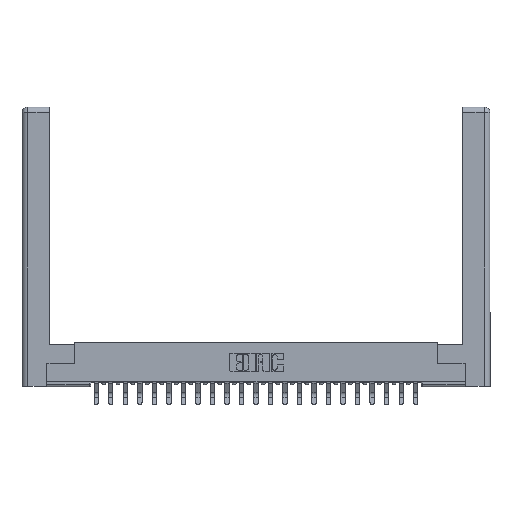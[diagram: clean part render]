
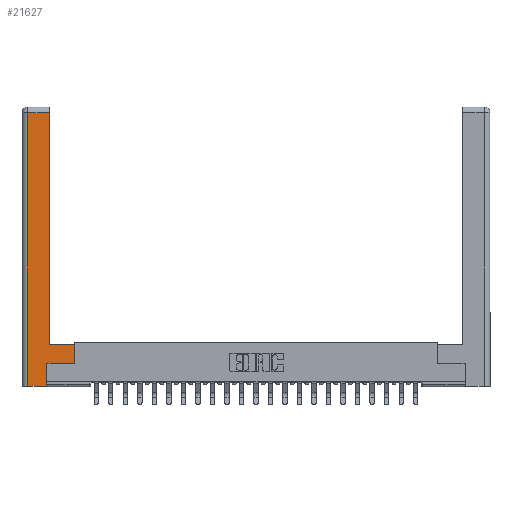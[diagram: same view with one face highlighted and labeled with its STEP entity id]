
A CAD part, top view. The second image highlights one B-rep face of the part: STEP entity #21627.
In plain terms, the highlighted planar face has unit normal (0, 0, 1).
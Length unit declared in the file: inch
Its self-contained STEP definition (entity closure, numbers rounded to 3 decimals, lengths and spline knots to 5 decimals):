
#479 = VECTOR ( 'NONE', #8831, 39.37008 ) ;
#528 = DIRECTION ( 'NONE',  ( -1., 0., 0. ) ) ;
#790 = CARTESIAN_POINT ( 'NONE',  ( 0., 0., 0. ) ) ;
#947 = CARTESIAN_POINT ( 'NONE',  ( 0.295, 0.45, 0. ) ) ;
#970 = CARTESIAN_POINT ( 'NONE',  ( 0.0615, 2.94, 0. ) ) ;
#2395 = EDGE_CURVE ( 'NONE', #10539, #5755, #22281, .T. ) ;
#3747 = DIRECTION ( 'NONE',  ( 0., -1., 0. ) ) ;
#3786 = AXIS2_PLACEMENT_3D ( 'NONE', #790, #4150, #8290 ) ;
#3849 = LINE ( 'NONE', #19378, #5885 ) ;
#4150 = DIRECTION ( 'NONE',  ( 0., 0., -1. ) ) ;
#4248 = VECTOR ( 'NONE', #17284, 39.37008 ) ;
#4791 = ORIENTED_EDGE ( 'NONE', *, *, #8718, .T. ) ;
#5755 = VERTEX_POINT ( 'NONE', #18787 ) ;
#5834 = EDGE_CURVE ( 'NONE', #10818, #13471, #13202, .T. ) ;
#5885 = VECTOR ( 'NONE', #7604, 39.37008 ) ;
#5921 = CARTESIAN_POINT ( 'NONE',  ( 0.265, 0.245, 0. ) ) ;
#6320 = VECTOR ( 'NONE', #3747, 39.37008 ) ;
#6873 = CARTESIAN_POINT ( 'NONE',  ( 0.565, 0.245, 0. ) ) ;
#6990 = CARTESIAN_POINT ( 'NONE',  ( 0.0615, 0., 0. ) ) ;
#7055 = EDGE_CURVE ( 'NONE', #21969, #10818, #14523, .T. ) ;
#7392 = CARTESIAN_POINT ( 'NONE',  ( 0.295, 3., 0. ) ) ;
#7604 = DIRECTION ( 'NONE',  ( 0., 1., 0. ) ) ;
#7853 = CARTESIAN_POINT ( 'NONE',  ( 0.295, 2.94, 0. ) ) ;
#8290 = DIRECTION ( 'NONE',  ( -1., 0., 0. ) ) ;
#8718 = EDGE_CURVE ( 'NONE', #19921, #14052, #13835, .T. ) ;
#8831 = DIRECTION ( 'NONE',  ( -1., 0., 0. ) ) ;
#9081 = VECTOR ( 'NONE', #24470, 39.37008 ) ;
#9848 = CARTESIAN_POINT ( 'NONE',  ( 0.265, 0., 0. ) ) ;
#10524 = VECTOR ( 'NONE', #528, 39.37008 ) ;
#10539 = VERTEX_POINT ( 'NONE', #5921 ) ;
#10818 = VERTEX_POINT ( 'NONE', #12743 ) ;
#11491 = ORIENTED_EDGE ( 'NONE', *, *, #15082, .T. ) ;
#11740 = CARTESIAN_POINT ( 'NONE',  ( 0.265, 0.245, 0. ) ) ;
#12139 = ORIENTED_EDGE ( 'NONE', *, *, #22338, .T. ) ;
#12413 = FACE_OUTER_BOUND ( 'NONE', #16506, .T. ) ;
#12743 = CARTESIAN_POINT ( 'NONE',  ( 0.295, 0.45, 0. ) ) ;
#13202 = LINE ( 'NONE', #7392, #20375 ) ;
#13386 = EDGE_CURVE ( 'NONE', #5755, #21969, #3849, .T. ) ;
#13471 = VERTEX_POINT ( 'NONE', #7853 ) ;
#13525 = LINE ( 'NONE', #11740, #4248 ) ;
#13835 = LINE ( 'NONE', #25347, #6320 ) ;
#14052 = VERTEX_POINT ( 'NONE', #6990 ) ;
#14523 = LINE ( 'NONE', #947, #479 ) ;
#15082 = EDGE_CURVE ( 'NONE', #14052, #18742, #19224, .T. ) ;
#16424 = PLANE ( 'NONE',  #3786 ) ;
#16506 = EDGE_LOOP ( 'NONE', ( #17088, #24292, #4791, #11491, #12139, #25166, #24618, #20090 ) ) ;
#17088 = ORIENTED_EDGE ( 'NONE', *, *, #5834, .T. ) ;
#17190 = CARTESIAN_POINT ( 'NONE',  ( 0.565, 0.45, 0. ) ) ;
#17284 = DIRECTION ( 'NONE',  ( 0., 1., 0. ) ) ;
#17390 = CARTESIAN_POINT ( 'NONE',  ( 0.265, 0., 0. ) ) ;
#17661 = DIRECTION ( 'NONE',  ( 1., 0., 0. ) ) ;
#18742 = VERTEX_POINT ( 'NONE', #9848 ) ;
#18787 = CARTESIAN_POINT ( 'NONE',  ( 0.565, 0.245, 0. ) ) ;
#19224 = LINE ( 'NONE', #17390, #24891 ) ;
#19304 = DIRECTION ( 'NONE',  ( 0., 1., 0. ) ) ;
#19378 = CARTESIAN_POINT ( 'NONE',  ( 0.565, 0.45, 0. ) ) ;
#19921 = VERTEX_POINT ( 'NONE', #970 ) ;
#20090 = ORIENTED_EDGE ( 'NONE', *, *, #7055, .T. ) ;
#20375 = VECTOR ( 'NONE', #19304, 39.37008 ) ;
#21627 = ADVANCED_FACE ( 'NONE', ( #12413 ), #16424, .F. ) ;
#21969 = VERTEX_POINT ( 'NONE', #17190 ) ;
#22139 = LINE ( 'NONE', #22257, #10524 ) ;
#22257 = CARTESIAN_POINT ( 'NONE',  ( 0.0615, 2.94, 0. ) ) ;
#22281 = LINE ( 'NONE', #6873, #9081 ) ;
#22338 = EDGE_CURVE ( 'NONE', #18742, #10539, #13525, .T. ) ;
#24292 = ORIENTED_EDGE ( 'NONE', *, *, #24572, .T. ) ;
#24470 = DIRECTION ( 'NONE',  ( 1., 0., 0. ) ) ;
#24572 = EDGE_CURVE ( 'NONE', #13471, #19921, #22139, .T. ) ;
#24618 = ORIENTED_EDGE ( 'NONE', *, *, #13386, .T. ) ;
#24891 = VECTOR ( 'NONE', #17661, 39.37008 ) ;
#25166 = ORIENTED_EDGE ( 'NONE', *, *, #2395, .T. ) ;
#25347 = CARTESIAN_POINT ( 'NONE',  ( 0.0615, 0., 0. ) ) ;
